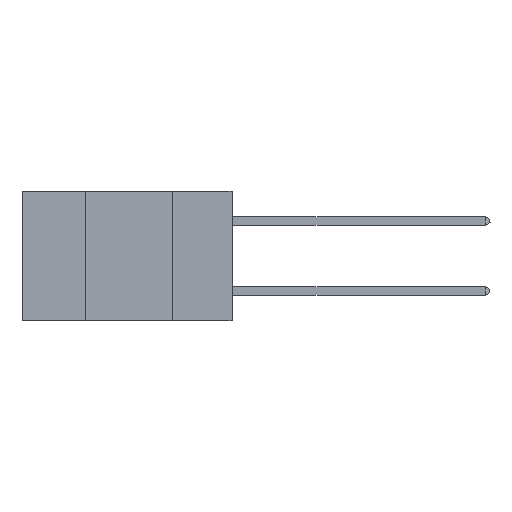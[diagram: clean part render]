
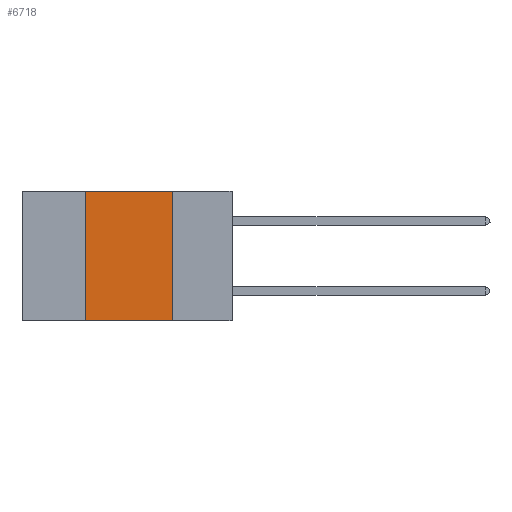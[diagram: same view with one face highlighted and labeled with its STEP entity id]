
A CAD part, left-side view. The second image highlights one B-rep face of the part: STEP entity #6718.
In plain terms, the highlighted planar face has unit normal (-1, 0, 0).
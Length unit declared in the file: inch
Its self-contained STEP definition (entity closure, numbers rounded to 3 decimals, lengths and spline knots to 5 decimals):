
#122 = LINE ( 'NONE', #17071, #7400 ) ;
#6219 = VECTOR ( 'NONE', #8770, 39.37008 ) ;
#6718 = ADVANCED_FACE ( 'NONE', ( #34957 ), #9685, .F. ) ;
#7400 = VECTOR ( 'NONE', #23347, 39.37008 ) ;
#8770 = DIRECTION ( 'NONE',  ( 0., 0., -1. ) ) ;
#9533 = DIRECTION ( 'NONE',  ( 0., 0., -1. ) ) ;
#9618 = VERTEX_POINT ( 'NONE', #23247 ) ;
#9685 = PLANE ( 'NONE',  #30396 ) ;
#10095 = CARTESIAN_POINT ( 'NONE',  ( 0., 0.42, 0. ) ) ;
#11921 = ORIENTED_EDGE ( 'NONE', *, *, #39648, .F. ) ;
#12254 = CARTESIAN_POINT ( 'NONE',  ( 0., 0.17, 0. ) ) ;
#15240 = EDGE_CURVE ( 'NONE', #9618, #35907, #15290, .T. ) ;
#15290 = LINE ( 'NONE', #29896, #15813 ) ;
#15460 = CARTESIAN_POINT ( 'NONE',  ( 0., 0.17, 0. ) ) ;
#15813 = VECTOR ( 'NONE', #39929, 39.37008 ) ;
#16947 = VECTOR ( 'NONE', #28265, 39.37008 ) ;
#17071 = CARTESIAN_POINT ( 'NONE',  ( 0., 0.6, 0. ) ) ;
#21231 = CARTESIAN_POINT ( 'NONE',  ( 0., 0.17, -0.37 ) ) ;
#21876 = DIRECTION ( 'NONE',  ( 1., 0., 0. ) ) ;
#23247 = CARTESIAN_POINT ( 'NONE',  ( 0., 0.42, -0.37 ) ) ;
#23347 = DIRECTION ( 'NONE',  ( 0., -1., 0. ) ) ;
#23907 = ORIENTED_EDGE ( 'NONE', *, *, #39726, .F. ) ;
#25753 = LINE ( 'NONE', #15460, #6219 ) ;
#28265 = DIRECTION ( 'NONE',  ( 0., 0., 1. ) ) ;
#28955 = EDGE_LOOP ( 'NONE', ( #11921, #33047, #23907, #34073 ) ) ;
#29896 = CARTESIAN_POINT ( 'NONE',  ( 0., 0.6, -0.37 ) ) ;
#30396 = AXIS2_PLACEMENT_3D ( 'NONE', #31504, #21876, #9533 ) ;
#30970 = VERTEX_POINT ( 'NONE', #10095 ) ;
#31504 = CARTESIAN_POINT ( 'NONE',  ( 0., 0.6, 0. ) ) ;
#31568 = VERTEX_POINT ( 'NONE', #12254 ) ;
#31663 = CARTESIAN_POINT ( 'NONE',  ( 0., 0.42, 0. ) ) ;
#33047 = ORIENTED_EDGE ( 'NONE', *, *, #33567, .F. ) ;
#33567 = EDGE_CURVE ( 'NONE', #30970, #31568, #122, .T. ) ;
#34073 = ORIENTED_EDGE ( 'NONE', *, *, #15240, .T. ) ;
#34448 = LINE ( 'NONE', #31663, #16947 ) ;
#34957 = FACE_OUTER_BOUND ( 'NONE', #28955, .T. ) ;
#35907 = VERTEX_POINT ( 'NONE', #21231 ) ;
#39648 = EDGE_CURVE ( 'NONE', #31568, #35907, #25753, .T. ) ;
#39726 = EDGE_CURVE ( 'NONE', #9618, #30970, #34448, .T. ) ;
#39929 = DIRECTION ( 'NONE',  ( 0., -1., 0. ) ) ;
